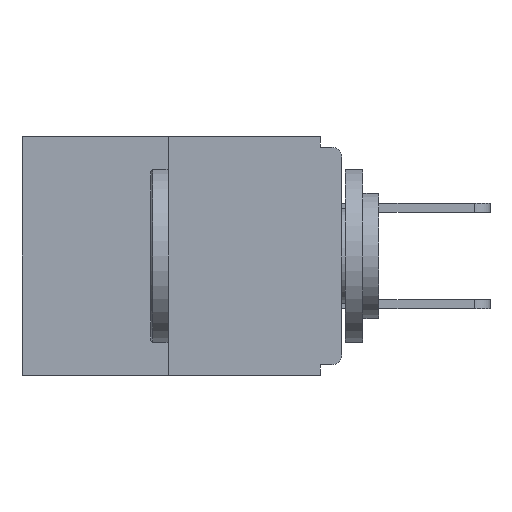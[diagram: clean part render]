
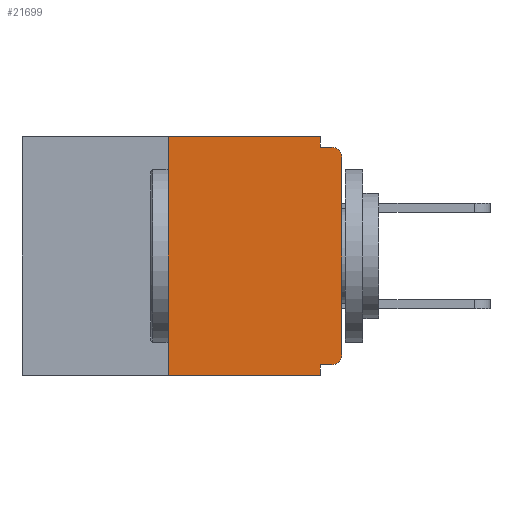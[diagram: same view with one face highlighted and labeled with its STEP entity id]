
A CAD part, left-side view. The second image highlights one B-rep face of the part: STEP entity #21699.
In plain terms, the highlighted planar face has unit normal (-1, 0, 0).
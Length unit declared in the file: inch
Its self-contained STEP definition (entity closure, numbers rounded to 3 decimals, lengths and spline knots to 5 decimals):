
#325 = VECTOR ( 'NONE', #15041, 39.37008 ) ;
#367 = ORIENTED_EDGE ( 'NONE', *, *, #3773, .T. ) ;
#944 = VERTEX_POINT ( 'NONE', #18182 ) ;
#1045 = LINE ( 'NONE', #1992, #14580 ) ;
#1635 = VECTOR ( 'NONE', #3179, 39.37008 ) ;
#1727 = EDGE_CURVE ( 'NONE', #6583, #12122, #12451, .T. ) ;
#1734 = EDGE_CURVE ( 'NONE', #21572, #12591, #14119, .T. ) ;
#1741 = CARTESIAN_POINT ( 'NONE',  ( 0., 0.46, 0. ) ) ;
#1913 = VECTOR ( 'NONE', #16155, 39.37008 ) ;
#1992 = CARTESIAN_POINT ( 'NONE',  ( 0., 0.46, -0.343 ) ) ;
#2061 = DIRECTION ( 'NONE',  ( -1., 0., 0. ) ) ;
#2231 = DIRECTION ( 'NONE',  ( 0., 1., 0. ) ) ;
#2468 = FACE_OUTER_BOUND ( 'NONE', #5891, .T. ) ;
#2540 = CARTESIAN_POINT ( 'NONE',  ( 0., 0., 0. ) ) ;
#2623 = CIRCLE ( 'NONE', #10629, 0.015 ) ;
#3009 = CARTESIAN_POINT ( 'NONE',  ( 0., 0.031, -0.343 ) ) ;
#3117 = CARTESIAN_POINT ( 'NONE',  ( 0., 0., -0.03 ) ) ;
#3179 = DIRECTION ( 'NONE',  ( 0., 0., -1. ) ) ;
#3346 = DIRECTION ( 'NONE',  ( 1., 0., 0. ) ) ;
#3755 = ORIENTED_EDGE ( 'NONE', *, *, #11091, .F. ) ;
#3773 = EDGE_CURVE ( 'NONE', #6583, #4995, #1045, .T. ) ;
#3798 = DIRECTION ( 'NONE',  ( 0., 0., -1. ) ) ;
#3956 = ORIENTED_EDGE ( 'NONE', *, *, #10604, .T. ) ;
#4085 = LINE ( 'NONE', #3009, #6922 ) ;
#4995 = VERTEX_POINT ( 'NONE', #17329 ) ;
#5049 = CARTESIAN_POINT ( 'NONE',  ( 0., 0.031, 0. ) ) ;
#5085 = CARTESIAN_POINT ( 'NONE',  ( 0., 0., -0.313 ) ) ;
#5891 = EDGE_LOOP ( 'NONE', ( #7899, #19734, #367, #7803, #17362, #14673, #7360, #3956, #3755, #14457 ) ) ;
#5986 = VECTOR ( 'NONE', #2231, 39.37008 ) ;
#6278 = CIRCLE ( 'NONE', #9533, 0.015 ) ;
#6373 = CARTESIAN_POINT ( 'NONE',  ( 0., 0.015, -0.328 ) ) ;
#6457 = LINE ( 'NONE', #6681, #1635 ) ;
#6477 = DIRECTION ( 'NONE',  ( 0., 0., -1. ) ) ;
#6583 = VERTEX_POINT ( 'NONE', #7603 ) ;
#6681 = CARTESIAN_POINT ( 'NONE',  ( 0., 0.031, 0. ) ) ;
#6758 = CARTESIAN_POINT ( 'NONE',  ( 0., 0.46, 0. ) ) ;
#6922 = VECTOR ( 'NONE', #13858, 39.37008 ) ;
#7360 = ORIENTED_EDGE ( 'NONE', *, *, #16074, .T. ) ;
#7603 = CARTESIAN_POINT ( 'NONE',  ( 0., 0.25, -0.343 ) ) ;
#7803 = ORIENTED_EDGE ( 'NONE', *, *, #23259, .F. ) ;
#7899 = ORIENTED_EDGE ( 'NONE', *, *, #14690, .F. ) ;
#8594 = CARTESIAN_POINT ( 'NONE',  ( 0., 0.25, 0. ) ) ;
#9533 = AXIS2_PLACEMENT_3D ( 'NONE', #15498, #22787, #6477 ) ;
#9666 = LINE ( 'NONE', #21498, #22082 ) ;
#9804 = LINE ( 'NONE', #1741, #1913 ) ;
#10188 = VERTEX_POINT ( 'NONE', #3117 ) ;
#10604 = EDGE_CURVE ( 'NONE', #10188, #944, #2623, .T. ) ;
#10629 = AXIS2_PLACEMENT_3D ( 'NONE', #18227, #2061, #3798 ) ;
#10886 = LINE ( 'NONE', #2540, #20721 ) ;
#11091 = EDGE_CURVE ( 'NONE', #20852, #944, #9666, .T. ) ;
#11649 = VERTEX_POINT ( 'NONE', #5085 ) ;
#12122 = VERTEX_POINT ( 'NONE', #8594 ) ;
#12235 = DIRECTION ( 'NONE',  ( 0., 0., 1. ) ) ;
#12344 = PLANE ( 'NONE',  #21818 ) ;
#12451 = LINE ( 'NONE', #14810, #325 ) ;
#12591 = VERTEX_POINT ( 'NONE', #21165 ) ;
#13019 = CARTESIAN_POINT ( 'NONE',  ( 0., 0., -0.328 ) ) ;
#13858 = DIRECTION ( 'NONE',  ( 0., 0., -1. ) ) ;
#13963 = DIRECTION ( 'NONE',  ( 0., 0., -1. ) ) ;
#14119 = LINE ( 'NONE', #13019, #5986 ) ;
#14457 = ORIENTED_EDGE ( 'NONE', *, *, #21651, .F. ) ;
#14497 = DIRECTION ( 'NONE',  ( 0., -1., 0. ) ) ;
#14580 = VECTOR ( 'NONE', #14497, 39.37008 ) ;
#14673 = ORIENTED_EDGE ( 'NONE', *, *, #18974, .T. ) ;
#14690 = EDGE_CURVE ( 'NONE', #12122, #17378, #9804, .T. ) ;
#14810 = CARTESIAN_POINT ( 'NONE',  ( 0., 0.25, 0. ) ) ;
#15041 = DIRECTION ( 'NONE',  ( 0., 0., 1. ) ) ;
#15498 = CARTESIAN_POINT ( 'NONE',  ( 0., 0.015, -0.313 ) ) ;
#16074 = EDGE_CURVE ( 'NONE', #11649, #10188, #10886, .T. ) ;
#16155 = DIRECTION ( 'NONE',  ( 0., -1., 0. ) ) ;
#17329 = CARTESIAN_POINT ( 'NONE',  ( 0., 0.031, -0.343 ) ) ;
#17362 = ORIENTED_EDGE ( 'NONE', *, *, #1734, .F. ) ;
#17378 = VERTEX_POINT ( 'NONE', #5049 ) ;
#17932 = DIRECTION ( 'NONE',  ( 0., -1., 0. ) ) ;
#18182 = CARTESIAN_POINT ( 'NONE',  ( 0., 0.015, -0.015 ) ) ;
#18227 = CARTESIAN_POINT ( 'NONE',  ( 0., 0.015, -0.03 ) ) ;
#18974 = EDGE_CURVE ( 'NONE', #21572, #11649, #6278, .T. ) ;
#19734 = ORIENTED_EDGE ( 'NONE', *, *, #1727, .F. ) ;
#20315 = CARTESIAN_POINT ( 'NONE',  ( 0., 0.031, -0.015 ) ) ;
#20721 = VECTOR ( 'NONE', #12235, 39.37008 ) ;
#20852 = VERTEX_POINT ( 'NONE', #20315 ) ;
#21165 = CARTESIAN_POINT ( 'NONE',  ( 0., 0.031, -0.328 ) ) ;
#21498 = CARTESIAN_POINT ( 'NONE',  ( 0., 0., -0.015 ) ) ;
#21572 = VERTEX_POINT ( 'NONE', #6373 ) ;
#21651 = EDGE_CURVE ( 'NONE', #17378, #20852, #6457, .T. ) ;
#21699 = ADVANCED_FACE ( 'NONE', ( #2468 ), #12344, .F. ) ;
#21818 = AXIS2_PLACEMENT_3D ( 'NONE', #6758, #3346, #13963 ) ;
#22082 = VECTOR ( 'NONE', #17932, 39.37008 ) ;
#22787 = DIRECTION ( 'NONE',  ( -1., 0., 0. ) ) ;
#23259 = EDGE_CURVE ( 'NONE', #12591, #4995, #4085, .T. ) ;
